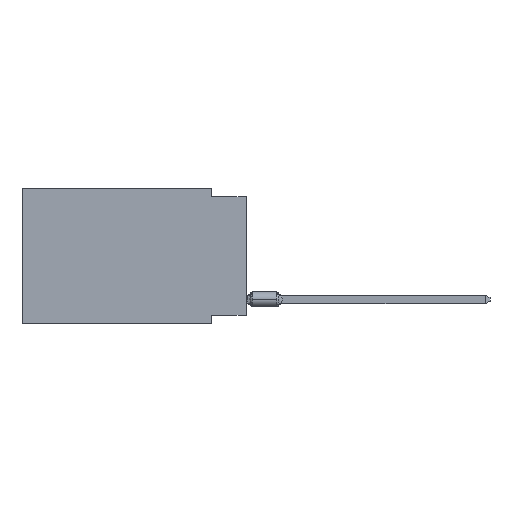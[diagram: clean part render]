
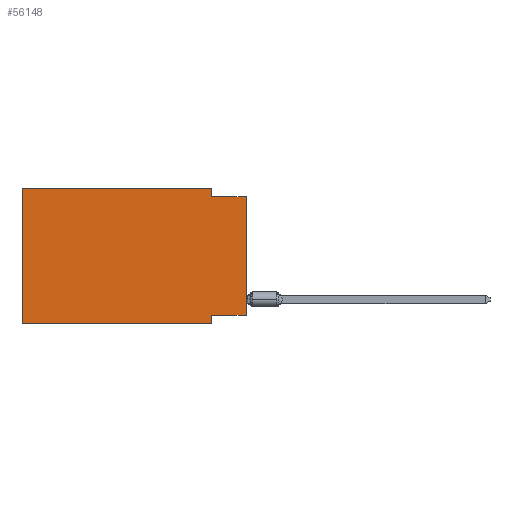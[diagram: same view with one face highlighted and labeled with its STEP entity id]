
A CAD part, left-side view. The second image highlights one B-rep face of the part: STEP entity #56148.
In plain terms, the highlighted planar face has unit normal (-1, 0, 0).
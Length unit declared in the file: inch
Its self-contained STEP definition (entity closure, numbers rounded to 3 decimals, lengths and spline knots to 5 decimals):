
#121 = VECTOR ( 'NONE', #47399, 39.37008 ) ;
#181 = ORIENTED_EDGE ( 'NONE', *, *, #40485, .F. ) ;
#685 = ORIENTED_EDGE ( 'NONE', *, *, #40019, .T. ) ;
#1746 = DIRECTION ( 'NONE',  ( 0., -1., 0. ) ) ;
#4196 = VERTEX_POINT ( 'NONE', #7483 ) ;
#4686 = ORIENTED_EDGE ( 'NONE', *, *, #37057, .F. ) ;
#4929 = VECTOR ( 'NONE', #7677, 39.37008 ) ;
#5603 = CARTESIAN_POINT ( 'NONE',  ( 0., 0.1, 0. ) ) ;
#6196 = CARTESIAN_POINT ( 'NONE',  ( 0., 0.645, 0. ) ) ;
#6731 = LINE ( 'NONE', #21790, #18881 ) ;
#7239 = VERTEX_POINT ( 'NONE', #26136 ) ;
#7483 = CARTESIAN_POINT ( 'NONE',  ( 0., 0., -0.025 ) ) ;
#7677 = DIRECTION ( 'NONE',  ( 0., 0., -1. ) ) ;
#9189 = LINE ( 'NONE', #45113, #10887 ) ;
#10887 = VECTOR ( 'NONE', #30051, 39.37008 ) ;
#10994 = DIRECTION ( 'NONE',  ( 1., 0., 0. ) ) ;
#11371 = ORIENTED_EDGE ( 'NONE', *, *, #43047, .T. ) ;
#12156 = LINE ( 'NONE', #12840, #4929 ) ;
#12840 = CARTESIAN_POINT ( 'NONE',  ( 0., 0.1, -0.39 ) ) ;
#13694 = ORIENTED_EDGE ( 'NONE', *, *, #19015, .F. ) ;
#16145 = ORIENTED_EDGE ( 'NONE', *, *, #44895, .F. ) ;
#18881 = VECTOR ( 'NONE', #64495, 39.37008 ) ;
#19015 = EDGE_CURVE ( 'NONE', #43803, #7239, #47084, .T. ) ;
#19607 = ORIENTED_EDGE ( 'NONE', *, *, #60477, .F. ) ;
#20927 = PLANE ( 'NONE',  #34623 ) ;
#21790 = CARTESIAN_POINT ( 'NONE',  ( 0., 0., 0. ) ) ;
#22576 = CARTESIAN_POINT ( 'NONE',  ( 0., 0.645, 0. ) ) ;
#22732 = VERTEX_POINT ( 'NONE', #22576 ) ;
#23628 = VERTEX_POINT ( 'NONE', #53190 ) ;
#25053 = VERTEX_POINT ( 'NONE', #45621 ) ;
#26136 = CARTESIAN_POINT ( 'NONE',  ( 0., 0.1, -0.025 ) ) ;
#26204 = LINE ( 'NONE', #42953, #121 ) ;
#30051 = DIRECTION ( 'NONE',  ( 0., -1., 0. ) ) ;
#32188 = FACE_OUTER_BOUND ( 'NONE', #39179, .T. ) ;
#32190 = VECTOR ( 'NONE', #35818, 39.37008 ) ;
#32210 = DIRECTION ( 'NONE',  ( 0., -1., 0. ) ) ;
#34536 = VERTEX_POINT ( 'NONE', #46401 ) ;
#34623 = AXIS2_PLACEMENT_3D ( 'NONE', #6196, #10994, #58479 ) ;
#35818 = DIRECTION ( 'NONE',  ( 0., 0., -1. ) ) ;
#36838 = CARTESIAN_POINT ( 'NONE',  ( 0., 0.1, 0. ) ) ;
#37057 = EDGE_CURVE ( 'NONE', #7239, #4196, #9189, .T. ) ;
#39179 = EDGE_LOOP ( 'NONE', ( #11371, #4686, #13694, #61483, #19607, #685, #16145, #181 ) ) ;
#40019 = EDGE_CURVE ( 'NONE', #34536, #25053, #58500, .T. ) ;
#40093 = VECTOR ( 'NONE', #1746, 39.37008 ) ;
#40485 = EDGE_CURVE ( 'NONE', #40742, #23628, #66157, .T. ) ;
#40742 = VERTEX_POINT ( 'NONE', #52811 ) ;
#42953 = CARTESIAN_POINT ( 'NONE',  ( 0., 0.645, 0. ) ) ;
#43047 = EDGE_CURVE ( 'NONE', #40742, #4196, #6731, .T. ) ;
#43803 = VERTEX_POINT ( 'NONE', #5603 ) ;
#44895 = EDGE_CURVE ( 'NONE', #23628, #25053, #12156, .T. ) ;
#45113 = CARTESIAN_POINT ( 'NONE',  ( 0., 0., -0.025 ) ) ;
#45621 = CARTESIAN_POINT ( 'NONE',  ( 0., 0.1, -0.39 ) ) ;
#46000 = CARTESIAN_POINT ( 'NONE',  ( 0., 0., -0.365 ) ) ;
#46401 = CARTESIAN_POINT ( 'NONE',  ( 0., 0.645, -0.39 ) ) ;
#47084 = LINE ( 'NONE', #36838, #32190 ) ;
#47399 = DIRECTION ( 'NONE',  ( 0., 0., 1. ) ) ;
#48570 = LINE ( 'NONE', #65885, #40093 ) ;
#52566 = VECTOR ( 'NONE', #66833, 39.37008 ) ;
#52811 = CARTESIAN_POINT ( 'NONE',  ( 0., 0., -0.365 ) ) ;
#53190 = CARTESIAN_POINT ( 'NONE',  ( 0., 0.1, -0.365 ) ) ;
#56148 = ADVANCED_FACE ( 'NONE', ( #32188 ), #20927, .F. ) ;
#56297 = EDGE_CURVE ( 'NONE', #22732, #43803, #48570, .T. ) ;
#57909 = VECTOR ( 'NONE', #32210, 39.37008 ) ;
#58168 = CARTESIAN_POINT ( 'NONE',  ( 0., 0.645, -0.39 ) ) ;
#58479 = DIRECTION ( 'NONE',  ( 0., 0., -1. ) ) ;
#58500 = LINE ( 'NONE', #58168, #57909 ) ;
#60477 = EDGE_CURVE ( 'NONE', #34536, #22732, #26204, .T. ) ;
#61483 = ORIENTED_EDGE ( 'NONE', *, *, #56297, .F. ) ;
#64495 = DIRECTION ( 'NONE',  ( 0., 0., 1. ) ) ;
#65885 = CARTESIAN_POINT ( 'NONE',  ( 0., 0.645, 0. ) ) ;
#66157 = LINE ( 'NONE', #46000, #52566 ) ;
#66833 = DIRECTION ( 'NONE',  ( 0., 1., 0. ) ) ;
